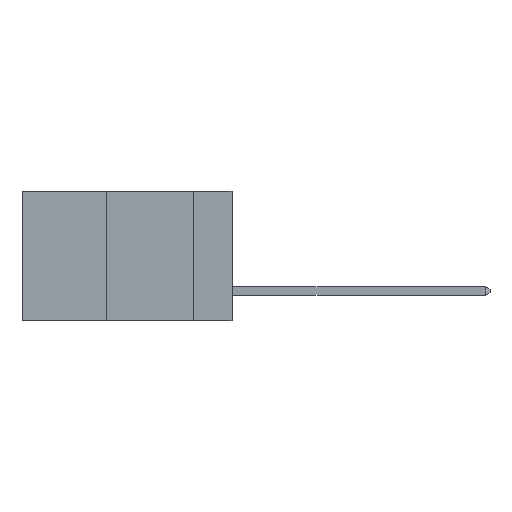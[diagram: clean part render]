
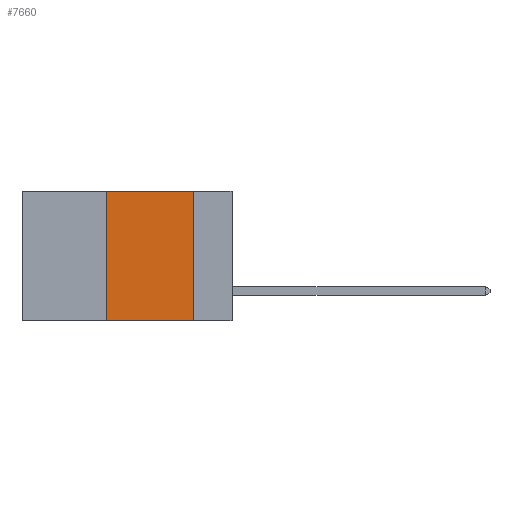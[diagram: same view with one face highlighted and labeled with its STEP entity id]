
A CAD part, left-side view. The second image highlights one B-rep face of the part: STEP entity #7660.
In plain terms, the highlighted planar face has unit normal (-1, 0, 0).
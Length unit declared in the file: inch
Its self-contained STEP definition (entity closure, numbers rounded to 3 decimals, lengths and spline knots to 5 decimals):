
#121 = DIRECTION ( 'NONE',  ( 1., 0., 0. ) ) ;
#829 = FACE_OUTER_BOUND ( 'NONE', #17234, .T. ) ;
#909 = VECTOR ( 'NONE', #13706, 39.37008 ) ;
#2295 = CARTESIAN_POINT ( 'NONE',  ( 0., 0.36, 0. ) ) ;
#2981 = VECTOR ( 'NONE', #10602, 39.37008 ) ;
#3821 = VECTOR ( 'NONE', #9695, 39.37008 ) ;
#3873 = CARTESIAN_POINT ( 'NONE',  ( 0., 0.36, 0. ) ) ;
#4685 = EDGE_CURVE ( 'NONE', #18085, #4772, #8751, .T. ) ;
#4772 = VERTEX_POINT ( 'NONE', #19538 ) ;
#5905 = CARTESIAN_POINT ( 'NONE',  ( 0., 0.36, -0.37 ) ) ;
#6368 = AXIS2_PLACEMENT_3D ( 'NONE', #8408, #121, #11832 ) ;
#6471 = CARTESIAN_POINT ( 'NONE',  ( 0., 0.6, -0.37 ) ) ;
#7522 = EDGE_CURVE ( 'NONE', #13019, #9661, #16619, .T. ) ;
#7660 = ADVANCED_FACE ( 'NONE', ( #829 ), #19769, .F. ) ;
#8144 = DIRECTION ( 'NONE',  ( 0., -1., 0. ) ) ;
#8408 = CARTESIAN_POINT ( 'NONE',  ( 0., 0.6, 0. ) ) ;
#8751 = LINE ( 'NONE', #17756, #3821 ) ;
#9335 = ORIENTED_EDGE ( 'NONE', *, *, #14155, .F. ) ;
#9377 = ORIENTED_EDGE ( 'NONE', *, *, #4685, .F. ) ;
#9640 = ORIENTED_EDGE ( 'NONE', *, *, #12951, .F. ) ;
#9661 = VERTEX_POINT ( 'NONE', #19130 ) ;
#9695 = DIRECTION ( 'NONE',  ( 0., -1., 0. ) ) ;
#10602 = DIRECTION ( 'NONE',  ( 0., 0., 1. ) ) ;
#11320 = ORIENTED_EDGE ( 'NONE', *, *, #7522, .T. ) ;
#11832 = DIRECTION ( 'NONE',  ( 0., 0., -1. ) ) ;
#12347 = LINE ( 'NONE', #3873, #2981 ) ;
#12951 = EDGE_CURVE ( 'NONE', #4772, #9661, #18378, .T. ) ;
#13019 = VERTEX_POINT ( 'NONE', #5905 ) ;
#13646 = CARTESIAN_POINT ( 'NONE',  ( 0., 0.11, 0. ) ) ;
#13706 = DIRECTION ( 'NONE',  ( 0., 0., -1. ) ) ;
#14155 = EDGE_CURVE ( 'NONE', #13019, #18085, #12347, .T. ) ;
#16117 = VECTOR ( 'NONE', #8144, 39.37008 ) ;
#16619 = LINE ( 'NONE', #6471, #16117 ) ;
#17234 = EDGE_LOOP ( 'NONE', ( #9640, #9377, #9335, #11320 ) ) ;
#17756 = CARTESIAN_POINT ( 'NONE',  ( 0., 0.6, 0. ) ) ;
#18085 = VERTEX_POINT ( 'NONE', #2295 ) ;
#18378 = LINE ( 'NONE', #13646, #909 ) ;
#19130 = CARTESIAN_POINT ( 'NONE',  ( 0., 0.11, -0.37 ) ) ;
#19538 = CARTESIAN_POINT ( 'NONE',  ( 0., 0.11, 0. ) ) ;
#19769 = PLANE ( 'NONE',  #6368 ) ;
